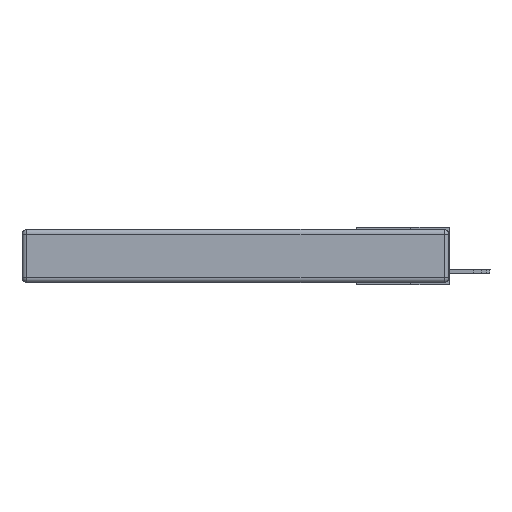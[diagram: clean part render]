
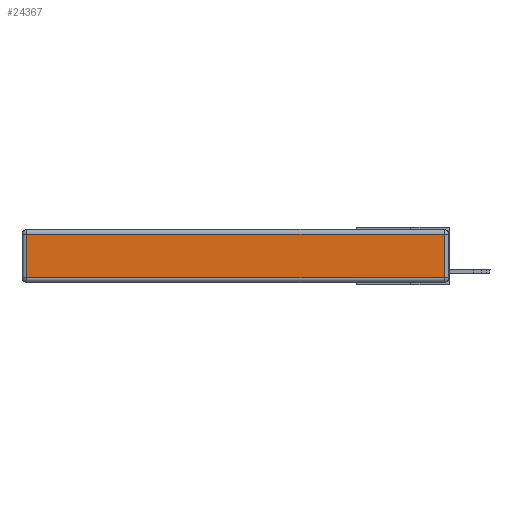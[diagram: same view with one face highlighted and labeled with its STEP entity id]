
A CAD part, left-side view. The second image highlights one B-rep face of the part: STEP entity #24367.
In plain terms, the highlighted planar face has unit normal (-1, 0, 0).
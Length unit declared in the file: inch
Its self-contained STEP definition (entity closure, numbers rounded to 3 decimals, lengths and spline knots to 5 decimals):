
#35 = VERTEX_POINT ( 'NONE', #26927 ) ;
#1296 = LINE ( 'NONE', #10391, #5985 ) ;
#2403 = ORIENTED_EDGE ( 'NONE', *, *, #20020, .T. ) ;
#2617 = DIRECTION ( 'NONE',  ( 0., 0., 1. ) ) ;
#4240 = CARTESIAN_POINT ( 'NONE',  ( 0., 0., -0.313 ) ) ;
#4517 = FACE_OUTER_BOUND ( 'NONE', #8919, .T. ) ;
#4812 = VECTOR ( 'NONE', #27780, 39.37008 ) ;
#5985 = VECTOR ( 'NONE', #21102, 39.37008 ) ;
#8166 = AXIS2_PLACEMENT_3D ( 'NONE', #15412, #26022, #2617 ) ;
#8181 = LINE ( 'NONE', #4240, #4812 ) ;
#8209 = CARTESIAN_POINT ( 'NONE',  ( 0., 2.72, -0.343 ) ) ;
#8919 = EDGE_LOOP ( 'NONE', ( #2403, #23732, #17476, #22817 ) ) ;
#10391 = CARTESIAN_POINT ( 'NONE',  ( 0., 2.75, -0.03 ) ) ;
#11132 = VERTEX_POINT ( 'NONE', #21490 ) ;
#12606 = LINE ( 'NONE', #8209, #23027 ) ;
#12793 = DIRECTION ( 'NONE',  ( 0., 0., -1. ) ) ;
#14349 = DIRECTION ( 'NONE',  ( 0., 0., 1. ) ) ;
#15233 = PLANE ( 'NONE',  #8166 ) ;
#15412 = CARTESIAN_POINT ( 'NONE',  ( 0., 0., -0.343 ) ) ;
#16704 = EDGE_CURVE ( 'NONE', #35, #27495, #1296, .T. ) ;
#17476 = ORIENTED_EDGE ( 'NONE', *, *, #16704, .T. ) ;
#17803 = EDGE_CURVE ( 'NONE', #18821, #35, #20695, .T. ) ;
#17960 = EDGE_CURVE ( 'NONE', #27495, #11132, #12606, .T. ) ;
#18821 = VERTEX_POINT ( 'NONE', #26467 ) ;
#19639 = CARTESIAN_POINT ( 'NONE',  ( 0., 2.72, -0.03 ) ) ;
#20020 = EDGE_CURVE ( 'NONE', #11132, #18821, #8181, .T. ) ;
#20695 = LINE ( 'NONE', #22603, #24349 ) ;
#21102 = DIRECTION ( 'NONE',  ( 0., 1., 0. ) ) ;
#21490 = CARTESIAN_POINT ( 'NONE',  ( 0., 2.72, -0.313 ) ) ;
#22603 = CARTESIAN_POINT ( 'NONE',  ( 0., 0.03, -0.343 ) ) ;
#22817 = ORIENTED_EDGE ( 'NONE', *, *, #17960, .T. ) ;
#23027 = VECTOR ( 'NONE', #12793, 39.37008 ) ;
#23732 = ORIENTED_EDGE ( 'NONE', *, *, #17803, .T. ) ;
#24349 = VECTOR ( 'NONE', #14349, 39.37008 ) ;
#24367 = ADVANCED_FACE ( 'NONE', ( #4517 ), #15233, .T. ) ;
#26022 = DIRECTION ( 'NONE',  ( -1., 0., 0. ) ) ;
#26467 = CARTESIAN_POINT ( 'NONE',  ( 0., 0.03, -0.313 ) ) ;
#26927 = CARTESIAN_POINT ( 'NONE',  ( 0., 0.03, -0.03 ) ) ;
#27495 = VERTEX_POINT ( 'NONE', #19639 ) ;
#27780 = DIRECTION ( 'NONE',  ( 0., -1., 0. ) ) ;
